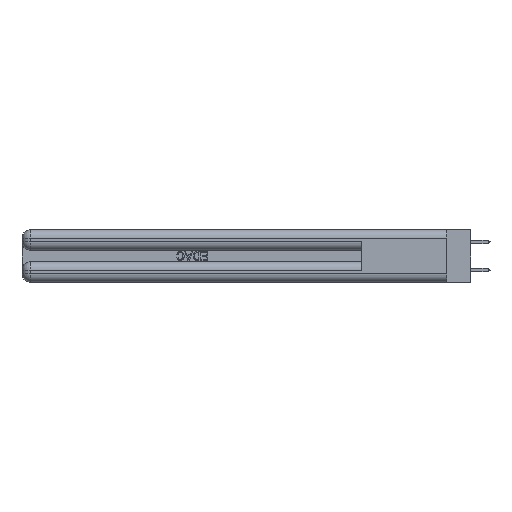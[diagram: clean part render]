
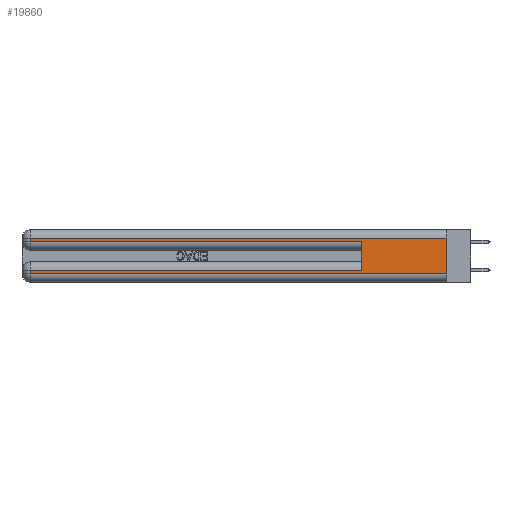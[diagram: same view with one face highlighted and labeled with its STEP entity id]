
A CAD part, left-side view. The second image highlights one B-rep face of the part: STEP entity #19860.
In plain terms, the highlighted planar face has unit normal (-1, 0, 0).
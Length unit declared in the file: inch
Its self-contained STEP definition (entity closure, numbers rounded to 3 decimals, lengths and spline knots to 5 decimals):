
#911 = VECTOR ( 'NONE', #18933, 39.37008 ) ;
#1308 = EDGE_CURVE ( 'NONE', #17490, #42732, #8669, .T. ) ;
#1901 = VERTEX_POINT ( 'NONE', #18340 ) ;
#3177 = CARTESIAN_POINT ( 'NONE',  ( 0., 2.94, 0.285 ) ) ;
#3245 = VERTEX_POINT ( 'NONE', #5894 ) ;
#3281 = DIRECTION ( 'NONE',  ( 0., -1., 0. ) ) ;
#3454 = VECTOR ( 'NONE', #19880, 39.37008 ) ;
#3780 = PLANE ( 'NONE',  #14990 ) ;
#3912 = CARTESIAN_POINT ( 'NONE',  ( 0., 0., 0.37 ) ) ;
#4979 = CARTESIAN_POINT ( 'NONE',  ( 0., 2.94, 0.085 ) ) ;
#5894 = CARTESIAN_POINT ( 'NONE',  ( 0., 0.6, 0.085 ) ) ;
#6138 = DIRECTION ( 'NONE',  ( 0., -1., 0. ) ) ;
#6276 = ORIENTED_EDGE ( 'NONE', *, *, #12735, .T. ) ;
#6551 = VECTOR ( 'NONE', #42483, 39.37008 ) ;
#6832 = VERTEX_POINT ( 'NONE', #37240 ) ;
#6944 = CARTESIAN_POINT ( 'NONE',  ( 0., 0.6, 0.145 ) ) ;
#7285 = DIRECTION ( 'NONE',  ( 1., 0., 0. ) ) ;
#8415 = CARTESIAN_POINT ( 'NONE',  ( 0., 2.94, 0.37 ) ) ;
#8669 = LINE ( 'NONE', #14484, #36553 ) ;
#8704 = LINE ( 'NONE', #38107, #41787 ) ;
#9265 = ORIENTED_EDGE ( 'NONE', *, *, #26854, .T. ) ;
#9905 = CARTESIAN_POINT ( 'NONE',  ( 0., 0., 0.085 ) ) ;
#10101 = VERTEX_POINT ( 'NONE', #3177 ) ;
#10423 = VECTOR ( 'NONE', #10673, 39.37008 ) ;
#10673 = DIRECTION ( 'NONE',  ( 0., 0., 1. ) ) ;
#10830 = LINE ( 'NONE', #8415, #911 ) ;
#11978 = LINE ( 'NONE', #27033, #34206 ) ;
#12735 = EDGE_CURVE ( 'NONE', #42732, #26078, #11978, .T. ) ;
#14484 = CARTESIAN_POINT ( 'NONE',  ( 0., 2.94, 0.37 ) ) ;
#14990 = AXIS2_PLACEMENT_3D ( 'NONE', #3912, #7285, #28278 ) ;
#16113 = ORIENTED_EDGE ( 'NONE', *, *, #26111, .T. ) ;
#17490 = VERTEX_POINT ( 'NONE', #4979 ) ;
#17951 = ORIENTED_EDGE ( 'NONE', *, *, #1308, .T. ) ;
#18150 = DIRECTION ( 'NONE',  ( 0., 1., 0. ) ) ;
#18340 = CARTESIAN_POINT ( 'NONE',  ( 0., 0.6, 0.285 ) ) ;
#18933 = DIRECTION ( 'NONE',  ( 0., 0., -1. ) ) ;
#19757 = LINE ( 'NONE', #6944, #10423 ) ;
#19860 = ADVANCED_FACE ( 'NONE', ( #29145 ), #3780, .F. ) ;
#19880 = DIRECTION ( 'NONE',  ( 0., 1., 0. ) ) ;
#20503 = LINE ( 'NONE', #36518, #6551 ) ;
#21474 = EDGE_CURVE ( 'NONE', #6832, #10101, #10830, .T. ) ;
#25538 = EDGE_LOOP ( 'NONE', ( #41003, #16113, #37162, #26688, #35575, #9265, #17951, #6276 ) ) ;
#26078 = VERTEX_POINT ( 'NONE', #41290 ) ;
#26111 = EDGE_CURVE ( 'NONE', #32586, #6832, #8704, .T. ) ;
#26688 = ORIENTED_EDGE ( 'NONE', *, *, #29788, .T. ) ;
#26854 = EDGE_CURVE ( 'NONE', #3245, #17490, #35538, .T. ) ;
#27033 = CARTESIAN_POINT ( 'NONE',  ( 0., 0., 0.06 ) ) ;
#27556 = DIRECTION ( 'NONE',  ( 0., 0., -1. ) ) ;
#28278 = DIRECTION ( 'NONE',  ( 0., 0., -1. ) ) ;
#29145 = FACE_OUTER_BOUND ( 'NONE', #25538, .T. ) ;
#29788 = EDGE_CURVE ( 'NONE', #10101, #1901, #41033, .T. ) ;
#32586 = VERTEX_POINT ( 'NONE', #36608 ) ;
#34206 = VECTOR ( 'NONE', #3281, 39.37008 ) ;
#34775 = CARTESIAN_POINT ( 'NONE',  ( 0., 2.94, 0.06 ) ) ;
#35538 = LINE ( 'NONE', #9905, #3454 ) ;
#35575 = ORIENTED_EDGE ( 'NONE', *, *, #42051, .F. ) ;
#35620 = CARTESIAN_POINT ( 'NONE',  ( 0., 0., 0.285 ) ) ;
#36518 = CARTESIAN_POINT ( 'NONE',  ( 0., 0., 0.37 ) ) ;
#36553 = VECTOR ( 'NONE', #27556, 39.37008 ) ;
#36608 = CARTESIAN_POINT ( 'NONE',  ( 0., 0., 0.31 ) ) ;
#37162 = ORIENTED_EDGE ( 'NONE', *, *, #21474, .T. ) ;
#37240 = CARTESIAN_POINT ( 'NONE',  ( 0., 2.94, 0.31 ) ) ;
#38107 = CARTESIAN_POINT ( 'NONE',  ( 0., 0., 0.31 ) ) ;
#39245 = EDGE_CURVE ( 'NONE', #32586, #26078, #20503, .T. ) ;
#39989 = VECTOR ( 'NONE', #6138, 39.37008 ) ;
#41003 = ORIENTED_EDGE ( 'NONE', *, *, #39245, .F. ) ;
#41033 = LINE ( 'NONE', #35620, #39989 ) ;
#41290 = CARTESIAN_POINT ( 'NONE',  ( 0., 0., 0.06 ) ) ;
#41787 = VECTOR ( 'NONE', #18150, 39.37008 ) ;
#42051 = EDGE_CURVE ( 'NONE', #3245, #1901, #19757, .T. ) ;
#42483 = DIRECTION ( 'NONE',  ( 0., 0., -1. ) ) ;
#42732 = VERTEX_POINT ( 'NONE', #34775 ) ;
